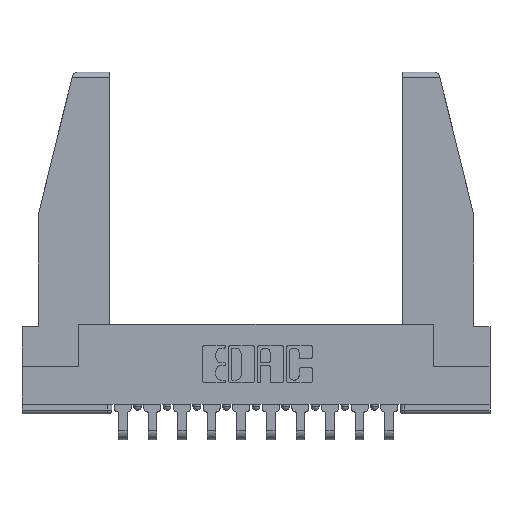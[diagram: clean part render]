
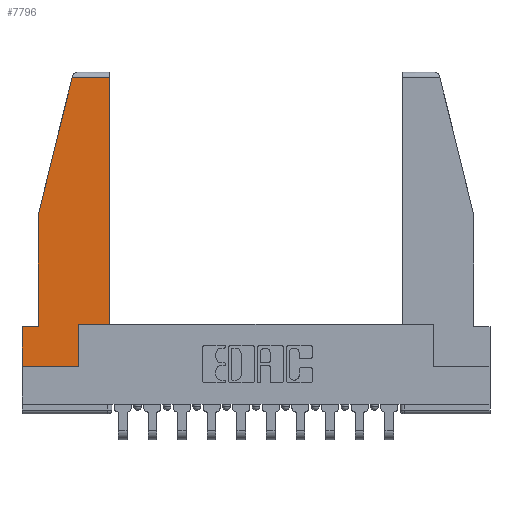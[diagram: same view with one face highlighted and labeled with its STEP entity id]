
A CAD part, top view. The second image highlights one B-rep face of the part: STEP entity #7796.
In plain terms, the highlighted planar face has unit normal (0, 0, 1).
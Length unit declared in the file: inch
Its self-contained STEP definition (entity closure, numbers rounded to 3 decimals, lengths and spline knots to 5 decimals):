
#92 = LINE ( 'NONE', #14102, #5774 ) ;
#230 = VERTEX_POINT ( 'NONE', #2988 ) ;
#253 = CARTESIAN_POINT ( 'NONE',  ( 0.086, 0.21, 0. ) ) ;
#434 = CARTESIAN_POINT ( 'NONE',  ( 0.297, 0., 0. ) ) ;
#509 = LINE ( 'NONE', #6873, #12492 ) ;
#681 = LINE ( 'NONE', #14955, #11597 ) ;
#752 = ORIENTED_EDGE ( 'NONE', *, *, #9397, .T. ) ;
#935 = LINE ( 'NONE', #12759, #4984 ) ;
#1012 = DIRECTION ( 'NONE',  ( -1., 0., 0. ) ) ;
#1120 = EDGE_CURVE ( 'NONE', #9899, #10608, #9186, .T. ) ;
#1133 = VERTEX_POINT ( 'NONE', #1623 ) ;
#1303 = VERTEX_POINT ( 'NONE', #5782 ) ;
#1367 = DIRECTION ( 'NONE',  ( 1., 0., 0. ) ) ;
#1598 = CARTESIAN_POINT ( 'NONE',  ( 0., 0., 0. ) ) ;
#1623 = CARTESIAN_POINT ( 'NONE',  ( 0.461, 1.52, 0. ) ) ;
#2115 = DIRECTION ( 'NONE',  ( 0., -1., 0. ) ) ;
#2133 = ORIENTED_EDGE ( 'NONE', *, *, #3756, .T. ) ;
#2145 = VECTOR ( 'NONE', #2115, 39.37008 ) ;
#2211 = LINE ( 'NONE', #3416, #7644 ) ;
#2375 = EDGE_CURVE ( 'NONE', #14979, #7268, #9669, .T. ) ;
#2430 = VECTOR ( 'NONE', #1012, 39.37008 ) ;
#2988 = CARTESIAN_POINT ( 'NONE',  ( 0.461, 0.223, 0. ) ) ;
#3416 = CARTESIAN_POINT ( 'NONE',  ( 0.297, 0., 0. ) ) ;
#3424 = VECTOR ( 'NONE', #9238, 39.37008 ) ;
#3756 = EDGE_CURVE ( 'NONE', #10608, #1303, #2211, .T. ) ;
#4241 = CARTESIAN_POINT ( 'NONE',  ( 0.461, 0.223, 0. ) ) ;
#4403 = CARTESIAN_POINT ( 'NONE',  ( 0., 0.21, 0. ) ) ;
#4416 = DIRECTION ( 'NONE',  ( -0.239, -0.971, 0. ) ) ;
#4486 = EDGE_CURVE ( 'NONE', #14168, #11470, #509, .T. ) ;
#4524 = ORIENTED_EDGE ( 'NONE', *, *, #14890, .T. ) ;
#4825 = EDGE_CURVE ( 'NONE', #7268, #9899, #681, .T. ) ;
#4984 = VECTOR ( 'NONE', #10480, 39.37008 ) ;
#5497 = ORIENTED_EDGE ( 'NONE', *, *, #1120, .T. ) ;
#5571 = CARTESIAN_POINT ( 'NONE',  ( 0.086, 0.8, 0. ) ) ;
#5739 = DIRECTION ( 'NONE',  ( 0., -1., 0. ) ) ;
#5774 = VECTOR ( 'NONE', #1367, 39.37008 ) ;
#5782 = CARTESIAN_POINT ( 'NONE',  ( 0.297, 0.223, 0. ) ) ;
#5826 = ORIENTED_EDGE ( 'NONE', *, *, #10448, .T. ) ;
#6260 = CARTESIAN_POINT ( 'NONE',  ( 0., 0., 0. ) ) ;
#6463 = LINE ( 'NONE', #4241, #3424 ) ;
#6638 = VECTOR ( 'NONE', #12662, 39.37008 ) ;
#6873 = CARTESIAN_POINT ( 'NONE',  ( 0.271, 1.55, 0. ) ) ;
#7095 = ORIENTED_EDGE ( 'NONE', *, *, #10038, .T. ) ;
#7268 = VERTEX_POINT ( 'NONE', #11263 ) ;
#7398 = AXIS2_PLACEMENT_3D ( 'NONE', #12657, #13799, #10247 ) ;
#7641 = EDGE_LOOP ( 'NONE', ( #7095, #4524, #9427, #752, #10525, #11852, #5497, #2133, #5826 ) ) ;
#7644 = VECTOR ( 'NONE', #12725, 39.37008 ) ;
#7796 = ADVANCED_FACE ( 'NONE', ( #13074 ), #9065, .T. ) ;
#8330 = LINE ( 'NONE', #5571, #2145 ) ;
#9065 = PLANE ( 'NONE',  #7398 ) ;
#9186 = LINE ( 'NONE', #1598, #6638 ) ;
#9238 = DIRECTION ( 'NONE',  ( 0., 1., 0. ) ) ;
#9397 = EDGE_CURVE ( 'NONE', #11470, #14979, #8330, .T. ) ;
#9427 = ORIENTED_EDGE ( 'NONE', *, *, #4486, .T. ) ;
#9669 = LINE ( 'NONE', #4403, #2430 ) ;
#9899 = VERTEX_POINT ( 'NONE', #6260 ) ;
#10038 = EDGE_CURVE ( 'NONE', #230, #1133, #6463, .T. ) ;
#10247 = DIRECTION ( 'NONE',  ( 1., 0., 0. ) ) ;
#10448 = EDGE_CURVE ( 'NONE', #1303, #230, #92, .T. ) ;
#10480 = DIRECTION ( 'NONE',  ( -1., 0., 0. ) ) ;
#10525 = ORIENTED_EDGE ( 'NONE', *, *, #2375, .T. ) ;
#10608 = VERTEX_POINT ( 'NONE', #434 ) ;
#11263 = CARTESIAN_POINT ( 'NONE',  ( 0., 0.21, 0. ) ) ;
#11470 = VERTEX_POINT ( 'NONE', #13475 ) ;
#11597 = VECTOR ( 'NONE', #5739, 39.37008 ) ;
#11852 = ORIENTED_EDGE ( 'NONE', *, *, #4825, .T. ) ;
#12492 = VECTOR ( 'NONE', #4416, 39.37008 ) ;
#12657 = CARTESIAN_POINT ( 'NONE',  ( 0., 0., 0. ) ) ;
#12662 = DIRECTION ( 'NONE',  ( 1., 0., 0. ) ) ;
#12718 = CARTESIAN_POINT ( 'NONE',  ( 0.2636, 1.52, 0. ) ) ;
#12725 = DIRECTION ( 'NONE',  ( 0., 1., 0. ) ) ;
#12759 = CARTESIAN_POINT ( 'NONE',  ( 0., 1.52, 0. ) ) ;
#13074 = FACE_OUTER_BOUND ( 'NONE', #7641, .T. ) ;
#13475 = CARTESIAN_POINT ( 'NONE',  ( 0.086, 0.8, 0. ) ) ;
#13799 = DIRECTION ( 'NONE',  ( 0., 0., 1. ) ) ;
#14102 = CARTESIAN_POINT ( 'NONE',  ( 0.297, 0.223, 0. ) ) ;
#14168 = VERTEX_POINT ( 'NONE', #12718 ) ;
#14890 = EDGE_CURVE ( 'NONE', #1133, #14168, #935, .T. ) ;
#14955 = CARTESIAN_POINT ( 'NONE',  ( 0., 0.21, 0. ) ) ;
#14979 = VERTEX_POINT ( 'NONE', #253 ) ;
